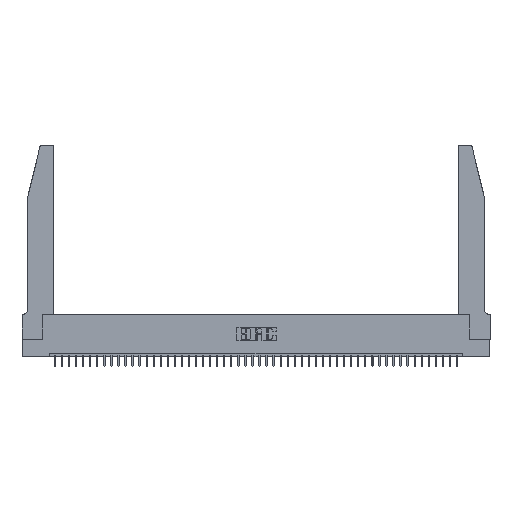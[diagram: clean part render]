
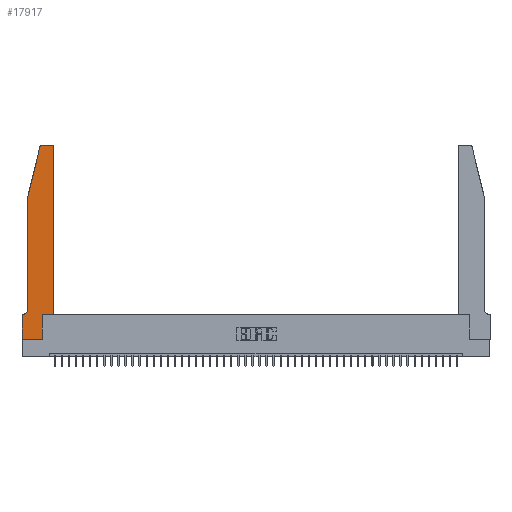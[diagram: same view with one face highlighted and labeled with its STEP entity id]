
A CAD part, top view. The second image highlights one B-rep face of the part: STEP entity #17917.
In plain terms, the highlighted planar face has unit normal (0, 0, 1).
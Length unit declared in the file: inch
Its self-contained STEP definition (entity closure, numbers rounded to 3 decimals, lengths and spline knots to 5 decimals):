
#40 = CARTESIAN_POINT ( 'NONE',  ( 0., 0., 0.37 ) ) ;
#567 = VERTEX_POINT ( 'NONE', #11440 ) ;
#832 = CARTESIAN_POINT ( 'NONE',  ( 0., 0., 0.37 ) ) ;
#1011 = ORIENTED_EDGE ( 'NONE', *, *, #5890, .T. ) ;
#1024 = DIRECTION ( 'NONE',  ( 0., -1., 0. ) ) ;
#1049 = VECTOR ( 'NONE', #44097, 39.37008 ) ;
#1213 = VECTOR ( 'NONE', #1024, 39.37008 ) ;
#1338 = EDGE_CURVE ( 'NONE', #24008, #12022, #37155, .T. ) ;
#1504 = CARTESIAN_POINT ( 'NONE',  ( 0.0755, 2., 0.37 ) ) ;
#2542 = ORIENTED_EDGE ( 'NONE', *, *, #11566, .T. ) ;
#2733 = CIRCLE ( 'NONE', #6631, 0.03 ) ;
#2745 = EDGE_CURVE ( 'NONE', #24868, #46867, #3529, .T. ) ;
#3410 = CARTESIAN_POINT ( 'NONE',  ( 0.0055, 0.35, 0.37 ) ) ;
#3529 = CIRCLE ( 'NONE', #47945, 0.07 ) ;
#4482 = CARTESIAN_POINT ( 'NONE',  ( 0.0755, 2., 0.37 ) ) ;
#4619 = DIRECTION ( 'NONE',  ( -1., 0., 0. ) ) ;
#4737 = LINE ( 'NONE', #28141, #23371 ) ;
#4790 = CARTESIAN_POINT ( 'NONE',  ( 0.4505, 0.35, 0.37 ) ) ;
#5693 = CARTESIAN_POINT ( 'NONE',  ( 0.4205, 2.75, 0.37 ) ) ;
#5890 = EDGE_CURVE ( 'NONE', #36002, #18564, #17968, .T. ) ;
#6118 = DIRECTION ( 'NONE',  ( -1., 0., 0. ) ) ;
#6631 = AXIS2_PLACEMENT_3D ( 'NONE', #41814, #15907, #8115 ) ;
#6691 = DIRECTION ( 'NONE',  ( 0., 0., 1. ) ) ;
#7326 = EDGE_CURVE ( 'NONE', #18985, #25520, #2733, .T. ) ;
#7425 = PLANE ( 'NONE',  #36246 ) ;
#8115 = DIRECTION ( 'NONE',  ( 1., 0., 0. ) ) ;
#8145 = VECTOR ( 'NONE', #45655, 39.37008 ) ;
#9917 = EDGE_LOOP ( 'NONE', ( #25920, #31294, #36401, #40057, #38957, #14603, #44796, #22417, #1011, #2542, #22619, #27001 ) ) ;
#9998 = VERTEX_POINT ( 'NONE', #4482 ) ;
#10120 = EDGE_CURVE ( 'NONE', #567, #12669, #37788, .T. ) ;
#10572 = EDGE_CURVE ( 'NONE', #9998, #24868, #27340, .T. ) ;
#11440 = CARTESIAN_POINT ( 'NONE',  ( 0.284, 2.75, 0.37 ) ) ;
#11566 = EDGE_CURVE ( 'NONE', #18564, #24631, #34829, .T. ) ;
#11744 = EDGE_CURVE ( 'NONE', #12022, #36002, #42627, .T. ) ;
#12022 = VERTEX_POINT ( 'NONE', #832 ) ;
#12612 = EDGE_CURVE ( 'NONE', #25520, #567, #31215, .T. ) ;
#12669 = VERTEX_POINT ( 'NONE', #13142 ) ;
#12968 = CARTESIAN_POINT ( 'NONE',  ( 0., 0.35, 0.37 ) ) ;
#13138 = CARTESIAN_POINT ( 'NONE',  ( 0.4505, 0.35, 0.37 ) ) ;
#13142 = CARTESIAN_POINT ( 'NONE',  ( 0.25487, 2.72718, 0.37 ) ) ;
#13395 = EDGE_CURVE ( 'NONE', #12669, #9998, #4737, .T. ) ;
#13658 = EDGE_CURVE ( 'NONE', #46867, #24008, #41080, .T. ) ;
#14603 = ORIENTED_EDGE ( 'NONE', *, *, #13658, .T. ) ;
#15907 = DIRECTION ( 'NONE',  ( 0., 0., 1. ) ) ;
#16176 = DIRECTION ( 'NONE',  ( 1., 0., 0. ) ) ;
#16481 = CARTESIAN_POINT ( 'NONE',  ( 0., 0., 0.37 ) ) ;
#16722 = DIRECTION ( 'NONE',  ( 1., 0., 0. ) ) ;
#16734 = AXIS2_PLACEMENT_3D ( 'NONE', #35474, #34997, #16176 ) ;
#17917 = ADVANCED_FACE ( 'NONE', ( #25229 ), #7425, .T. ) ;
#17968 = LINE ( 'NONE', #28489, #1049 ) ;
#18564 = VERTEX_POINT ( 'NONE', #31207 ) ;
#18985 = VERTEX_POINT ( 'NONE', #38960 ) ;
#21579 = DIRECTION ( 'NONE',  ( 1., 0., 0. ) ) ;
#22009 = VECTOR ( 'NONE', #33260, 39.37008 ) ;
#22207 = VECTOR ( 'NONE', #31507, 39.37008 ) ;
#22417 = ORIENTED_EDGE ( 'NONE', *, *, #11744, .T. ) ;
#22619 = ORIENTED_EDGE ( 'NONE', *, *, #22839, .T. ) ;
#22839 = EDGE_CURVE ( 'NONE', #24631, #18985, #42004, .T. ) ;
#23371 = VECTOR ( 'NONE', #28629, 39.37008 ) ;
#24008 = VERTEX_POINT ( 'NONE', #12968 ) ;
#24631 = VERTEX_POINT ( 'NONE', #13138 ) ;
#24646 = CARTESIAN_POINT ( 'NONE',  ( 0.0055, 0.42, 0.37 ) ) ;
#24868 = VERTEX_POINT ( 'NONE', #37507 ) ;
#25229 = FACE_OUTER_BOUND ( 'NONE', #9917, .T. ) ;
#25520 = VERTEX_POINT ( 'NONE', #5693 ) ;
#25920 = ORIENTED_EDGE ( 'NONE', *, *, #12612, .T. ) ;
#27001 = ORIENTED_EDGE ( 'NONE', *, *, #7326, .T. ) ;
#27340 = LINE ( 'NONE', #1504, #22207 ) ;
#27779 = CARTESIAN_POINT ( 'NONE',  ( 0.2605, 2.75, 0.37 ) ) ;
#28141 = CARTESIAN_POINT ( 'NONE',  ( 0.0755, 2., 0.37 ) ) ;
#28489 = CARTESIAN_POINT ( 'NONE',  ( 0.2865, 0.35, 0.37 ) ) ;
#28629 = DIRECTION ( 'NONE',  ( -0.239, -0.971, 0. ) ) ;
#28990 = VECTOR ( 'NONE', #16722, 39.37008 ) ;
#31207 = CARTESIAN_POINT ( 'NONE',  ( 0.2865, 0.35, 0.37 ) ) ;
#31215 = LINE ( 'NONE', #27779, #32181 ) ;
#31294 = ORIENTED_EDGE ( 'NONE', *, *, #10120, .T. ) ;
#31507 = DIRECTION ( 'NONE',  ( 0., -1., 0. ) ) ;
#32181 = VECTOR ( 'NONE', #4619, 39.37008 ) ;
#33260 = DIRECTION ( 'NONE',  ( -1., 0., 0. ) ) ;
#34829 = LINE ( 'NONE', #4790, #37567 ) ;
#34997 = DIRECTION ( 'NONE',  ( 0., 0., 1. ) ) ;
#35474 = CARTESIAN_POINT ( 'NONE',  ( 0.284, 2.72, 0.37 ) ) ;
#36002 = VERTEX_POINT ( 'NONE', #41099 ) ;
#36195 = CARTESIAN_POINT ( 'NONE',  ( 0.0755, 0.35, 0.37 ) ) ;
#36246 = AXIS2_PLACEMENT_3D ( 'NONE', #36954, #6691, #21579 ) ;
#36401 = ORIENTED_EDGE ( 'NONE', *, *, #13395, .T. ) ;
#36954 = CARTESIAN_POINT ( 'NONE',  ( 0., 0.35, 0.37 ) ) ;
#37155 = LINE ( 'NONE', #40, #1213 ) ;
#37507 = CARTESIAN_POINT ( 'NONE',  ( 0.0755, 0.42, 0.37 ) ) ;
#37567 = VECTOR ( 'NONE', #45803, 39.37008 ) ;
#37788 = CIRCLE ( 'NONE', #16734, 0.03 ) ;
#38082 = CARTESIAN_POINT ( 'NONE',  ( 0.4505, 0.35, 0.37 ) ) ;
#38957 = ORIENTED_EDGE ( 'NONE', *, *, #2745, .T. ) ;
#38960 = CARTESIAN_POINT ( 'NONE',  ( 0.4505, 2.72, 0.37 ) ) ;
#40057 = ORIENTED_EDGE ( 'NONE', *, *, #10572, .T. ) ;
#41080 = LINE ( 'NONE', #36195, #22009 ) ;
#41099 = CARTESIAN_POINT ( 'NONE',  ( 0.2865, 0., 0.37 ) ) ;
#41814 = CARTESIAN_POINT ( 'NONE',  ( 0.4205, 2.72, 0.37 ) ) ;
#42004 = LINE ( 'NONE', #38082, #8145 ) ;
#42627 = LINE ( 'NONE', #16481, #28990 ) ;
#44097 = DIRECTION ( 'NONE',  ( 0., 1., 0. ) ) ;
#44796 = ORIENTED_EDGE ( 'NONE', *, *, #1338, .T. ) ;
#45655 = DIRECTION ( 'NONE',  ( 0., 1., 0. ) ) ;
#45803 = DIRECTION ( 'NONE',  ( 1., 0., 0. ) ) ;
#45984 = DIRECTION ( 'NONE',  ( 0., 0., -1. ) ) ;
#46867 = VERTEX_POINT ( 'NONE', #3410 ) ;
#47945 = AXIS2_PLACEMENT_3D ( 'NONE', #24646, #45984, #6118 ) ;
